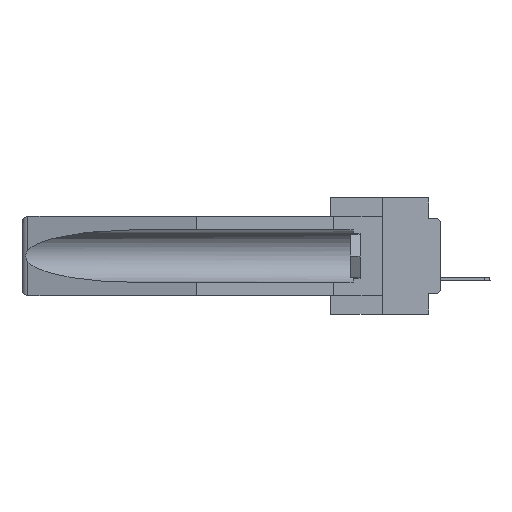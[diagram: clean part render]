
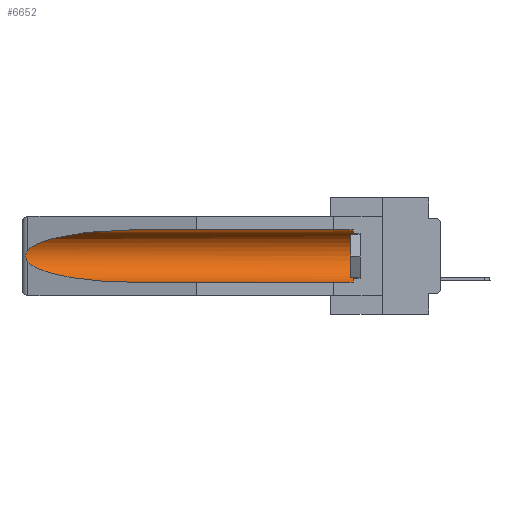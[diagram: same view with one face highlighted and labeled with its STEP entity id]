
A CAD part, left-side view. The second image highlights one B-rep face of the part: STEP entity #6652.
In plain terms, the highlighted cylindrical face has radius 2.857 mm (diameter 5.715 mm), a partial arc.
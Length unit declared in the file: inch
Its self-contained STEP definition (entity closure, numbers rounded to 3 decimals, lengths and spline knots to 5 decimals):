
#38 =( BOUNDED_CURVE ( )  B_SPLINE_CURVE ( 3, ( #26870, #35083, #3209, #8955 ),
 .UNSPECIFIED., .F., .F. ) 
 B_SPLINE_CURVE_WITH_KNOTS ( ( 4, 4 ),
 ( 4.71239, 6.08839 ),
 .UNSPECIFIED. ) 
 CURVE ( )  GEOMETRIC_REPRESENTATION_ITEM ( )  RATIONAL_B_SPLINE_CURVE ( ( 1., 0.848, 0.848, 1. ) ) 
 REPRESENTATION_ITEM ( '' )  );
#554 = ORIENTED_EDGE ( 'NONE', *, *, #14616, .F. ) ;
#645 = VERTEX_POINT ( 'NONE', #13284 ) ;
#1554 = B_SPLINE_CURVE_WITH_KNOTS ( 'NONE', 3,
 ( #25751, #10512, #13564, #37394, #28638, #4779, #19658, #31497, #10703, #27880 ),
 .UNSPECIFIED., .F., .F.,
 ( 4, 2, 2, 2, 4 ),
 ( 0., 0.00029, 0.00058, 0.00087, 0.00117 ),
 .UNSPECIFIED. ) ;
#1632 = CYLINDRICAL_SURFACE ( 'NONE', #30186, 0.1125 ) ;
#2956 = ORIENTED_EDGE ( 'NONE', *, *, #15454, .T. ) ;
#3209 = CARTESIAN_POINT ( 'NONE',  ( 0.25451, 1.48313, -0.09465 ) ) ;
#4438 = CARTESIAN_POINT ( 'NONE',  ( 0.155, 1.07973, -0.284 ) ) ;
#4444 = CARTESIAN_POINT ( 'NONE',  ( 0.155, 1.07973, -0.284 ) ) ;
#4779 = CARTESIAN_POINT ( 'NONE',  ( 0.2675, 1.53308, -0.17534 ) ) ;
#5235 = CIRCLE ( 'NONE', #10739, 0.1125 ) ;
#6026 = CARTESIAN_POINT ( 'NONE',  ( 0.155, -0.30754, -0.059 ) ) ;
#6047 = EDGE_CURVE ( 'NONE', #645, #13873, #38, .T. ) ;
#6114 = ORIENTED_EDGE ( 'NONE', *, *, #19164, .T. ) ;
#6143 = VERTEX_POINT ( 'NONE', #33545 ) ;
#6449 = VECTOR ( 'NONE', #37137, 39.37008 ) ;
#6652 = ADVANCED_FACE ( 'NONE', ( #27779 ), #1632, .F. ) ;
#8144 =( BOUNDED_CURVE ( )  B_SPLINE_CURVE ( 3, ( #37166, #18571, #24484, #4444 ),
 .UNSPECIFIED., .F., .F. ) 
 B_SPLINE_CURVE_WITH_KNOTS ( ( 4, 4 ),
 ( 0.1948, 1.5708 ),
 .UNSPECIFIED. ) 
 CURVE ( )  GEOMETRIC_REPRESENTATION_ITEM ( )  RATIONAL_B_SPLINE_CURVE ( ( 1., 0.848, 0.848, 1. ) ) 
 REPRESENTATION_ITEM ( '' )  );
#8955 = CARTESIAN_POINT ( 'NONE',  ( 0.26537, 1.52718, -0.14972 ) ) ;
#10370 = ORIENTED_EDGE ( 'NONE', *, *, #28143, .T. ) ;
#10512 = CARTESIAN_POINT ( 'NONE',  ( 0.26597, 1.52961, -0.15275 ) ) ;
#10703 = CARTESIAN_POINT ( 'NONE',  ( 0.26597, 1.5296, -0.19026 ) ) ;
#10739 = AXIS2_PLACEMENT_3D ( 'NONE', #14088, #11045, #22672 ) ;
#11045 = DIRECTION ( 'NONE',  ( 0., -1., 0. ) ) ;
#13284 = CARTESIAN_POINT ( 'NONE',  ( 0.155, 1.07973, -0.059 ) ) ;
#13325 = CARTESIAN_POINT ( 'NONE',  ( 0.155, 0.126, -0.059 ) ) ;
#13564 = CARTESIAN_POINT ( 'NONE',  ( 0.26654, 1.53092, -0.15636 ) ) ;
#13873 = VERTEX_POINT ( 'NONE', #33638 ) ;
#14088 = CARTESIAN_POINT ( 'NONE',  ( 0.155, 0.126, -0.1715 ) ) ;
#14616 = EDGE_CURVE ( 'NONE', #6143, #17731, #24197, .T. ) ;
#14740 = VERTEX_POINT ( 'NONE', #13325 ) ;
#15454 = EDGE_CURVE ( 'NONE', #13873, #37470, #1554, .T. ) ;
#15565 = CARTESIAN_POINT ( 'NONE',  ( 0.155, -0.30754, -0.1715 ) ) ;
#16686 = DIRECTION ( 'NONE',  ( 0., 0., 1. ) ) ;
#17182 = EDGE_CURVE ( 'NONE', #6143, #14740, #5235, .T. ) ;
#17731 = VERTEX_POINT ( 'NONE', #4438 ) ;
#18571 = CARTESIAN_POINT ( 'NONE',  ( 0.25451, 1.48313, -0.24835 ) ) ;
#19164 = EDGE_CURVE ( 'NONE', #37470, #17731, #8144, .T. ) ;
#19658 = CARTESIAN_POINT ( 'NONE',  ( 0.2673, 1.53269, -0.17917 ) ) ;
#20321 = EDGE_LOOP ( 'NONE', ( #31134, #2956, #6114, #554, #33181, #10370 ) ) ;
#20939 = VECTOR ( 'NONE', #32983, 39.37008 ) ;
#22207 = CARTESIAN_POINT ( 'NONE',  ( 0.26537, 1.52718, -0.19328 ) ) ;
#22672 = DIRECTION ( 'NONE',  ( 0., 0., 1. ) ) ;
#24197 = LINE ( 'NONE', #29556, #20939 ) ;
#24484 = CARTESIAN_POINT ( 'NONE',  ( 0.21114, 1.30732, -0.284 ) ) ;
#25751 = CARTESIAN_POINT ( 'NONE',  ( 0.26537, 1.52718, -0.14972 ) ) ;
#26870 = CARTESIAN_POINT ( 'NONE',  ( 0.155, 1.07973, -0.059 ) ) ;
#27210 = DIRECTION ( 'NONE',  ( 0., 1., 0. ) ) ;
#27779 = FACE_OUTER_BOUND ( 'NONE', #20321, .T. ) ;
#27880 = CARTESIAN_POINT ( 'NONE',  ( 0.26537, 1.52718, -0.19328 ) ) ;
#28143 = EDGE_CURVE ( 'NONE', #14740, #645, #35001, .T. ) ;
#28638 = CARTESIAN_POINT ( 'NONE',  ( 0.2675, 1.53308, -0.16763 ) ) ;
#29556 = CARTESIAN_POINT ( 'NONE',  ( 0.155, -0.30754, -0.284 ) ) ;
#30186 = AXIS2_PLACEMENT_3D ( 'NONE', #15565, #27210, #16686 ) ;
#31134 = ORIENTED_EDGE ( 'NONE', *, *, #6047, .T. ) ;
#31497 = CARTESIAN_POINT ( 'NONE',  ( 0.26655, 1.53094, -0.18657 ) ) ;
#32983 = DIRECTION ( 'NONE',  ( 0., 1., 0. ) ) ;
#33181 = ORIENTED_EDGE ( 'NONE', *, *, #17182, .T. ) ;
#33545 = CARTESIAN_POINT ( 'NONE',  ( 0.155, 0.126, -0.284 ) ) ;
#33638 = CARTESIAN_POINT ( 'NONE',  ( 0.26537, 1.52718, -0.14972 ) ) ;
#35001 = LINE ( 'NONE', #6026, #6449 ) ;
#35083 = CARTESIAN_POINT ( 'NONE',  ( 0.21114, 1.30732, -0.059 ) ) ;
#37137 = DIRECTION ( 'NONE',  ( 0., 1., 0. ) ) ;
#37166 = CARTESIAN_POINT ( 'NONE',  ( 0.26537, 1.52718, -0.19328 ) ) ;
#37394 = CARTESIAN_POINT ( 'NONE',  ( 0.2673, 1.5327, -0.16383 ) ) ;
#37470 = VERTEX_POINT ( 'NONE', #22207 ) ;
